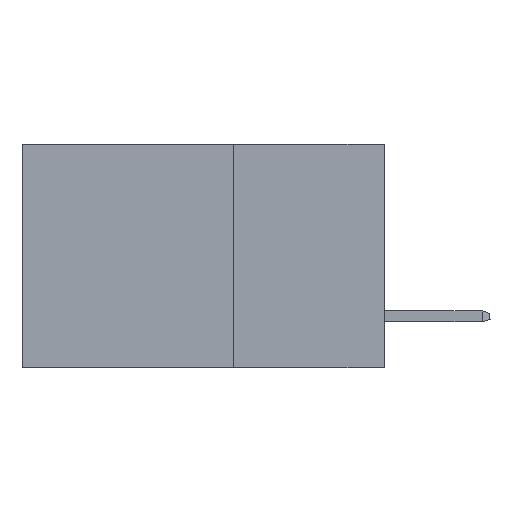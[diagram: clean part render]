
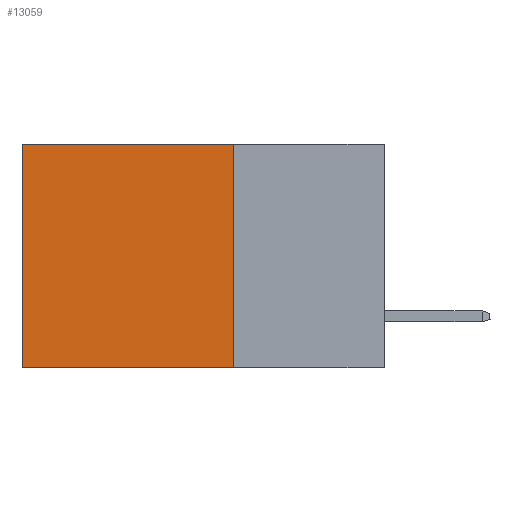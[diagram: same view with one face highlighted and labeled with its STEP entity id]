
A CAD part, left-side view. The second image highlights one B-rep face of the part: STEP entity #13059.
In plain terms, the highlighted planar face has unit normal (-1, 0, 0).
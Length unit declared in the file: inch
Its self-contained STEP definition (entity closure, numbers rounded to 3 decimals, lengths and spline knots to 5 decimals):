
#274 = PLANE ( 'NONE',  #9709 ) ;
#295 = CARTESIAN_POINT ( 'NONE',  ( 0.298, 0.6, -0.37 ) ) ;
#503 = DIRECTION ( 'NONE',  ( 0., 1., 0. ) ) ;
#1372 = DIRECTION ( 'NONE',  ( 0., 1., 0. ) ) ;
#1524 = ORIENTED_EDGE ( 'NONE', *, *, #14351, .F. ) ;
#1564 = CARTESIAN_POINT ( 'NONE',  ( 0.298, 0.25, 0. ) ) ;
#1624 = EDGE_CURVE ( 'NONE', #8912, #11017, #12134, .T. ) ;
#2863 = DIRECTION ( 'NONE',  ( 0., 0., -1. ) ) ;
#3565 = EDGE_CURVE ( 'NONE', #4268, #11017, #4861, .T. ) ;
#4268 = VERTEX_POINT ( 'NONE', #9911 ) ;
#4456 = DIRECTION ( 'NONE',  ( 0., 0., -1. ) ) ;
#4861 = LINE ( 'NONE', #5525, #5044 ) ;
#5044 = VECTOR ( 'NONE', #4456, 39.37008 ) ;
#5175 = LINE ( 'NONE', #9614, #13585 ) ;
#5525 = CARTESIAN_POINT ( 'NONE',  ( 0.298, 0.6, 0. ) ) ;
#6006 = DIRECTION ( 'NONE',  ( 0., 0., -1. ) ) ;
#7075 = DIRECTION ( 'NONE',  ( 1., 0., 0. ) ) ;
#7454 = ORIENTED_EDGE ( 'NONE', *, *, #3565, .T. ) ;
#7657 = VECTOR ( 'NONE', #1372, 39.37008 ) ;
#8536 = CARTESIAN_POINT ( 'NONE',  ( 0.298, 0.25, -0.37 ) ) ;
#8606 = LINE ( 'NONE', #1564, #12356 ) ;
#8912 = VERTEX_POINT ( 'NONE', #8536 ) ;
#9010 = FACE_OUTER_BOUND ( 'NONE', #12684, .T. ) ;
#9538 = EDGE_CURVE ( 'NONE', #11189, #4268, #5175, .T. ) ;
#9614 = CARTESIAN_POINT ( 'NONE',  ( 0.298, 0.25, 0. ) ) ;
#9709 = AXIS2_PLACEMENT_3D ( 'NONE', #13672, #7075, #6006 ) ;
#9911 = CARTESIAN_POINT ( 'NONE',  ( 0.298, 0.6, 0. ) ) ;
#9974 = CARTESIAN_POINT ( 'NONE',  ( 0.298, 0.25, -0.37 ) ) ;
#10600 = CARTESIAN_POINT ( 'NONE',  ( 0.298, 0.25, 0. ) ) ;
#11017 = VERTEX_POINT ( 'NONE', #295 ) ;
#11189 = VERTEX_POINT ( 'NONE', #10600 ) ;
#12111 = ORIENTED_EDGE ( 'NONE', *, *, #9538, .T. ) ;
#12134 = LINE ( 'NONE', #9974, #7657 ) ;
#12356 = VECTOR ( 'NONE', #2863, 39.37008 ) ;
#12684 = EDGE_LOOP ( 'NONE', ( #7454, #13681, #1524, #12111 ) ) ;
#13059 = ADVANCED_FACE ( 'NONE', ( #9010 ), #274, .F. ) ;
#13585 = VECTOR ( 'NONE', #503, 39.37008 ) ;
#13672 = CARTESIAN_POINT ( 'NONE',  ( 0.298, 0.25, 0. ) ) ;
#13681 = ORIENTED_EDGE ( 'NONE', *, *, #1624, .F. ) ;
#14351 = EDGE_CURVE ( 'NONE', #11189, #8912, #8606, .T. ) ;
